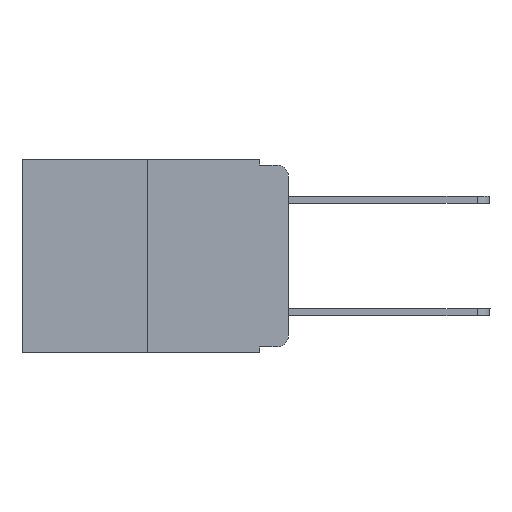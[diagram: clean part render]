
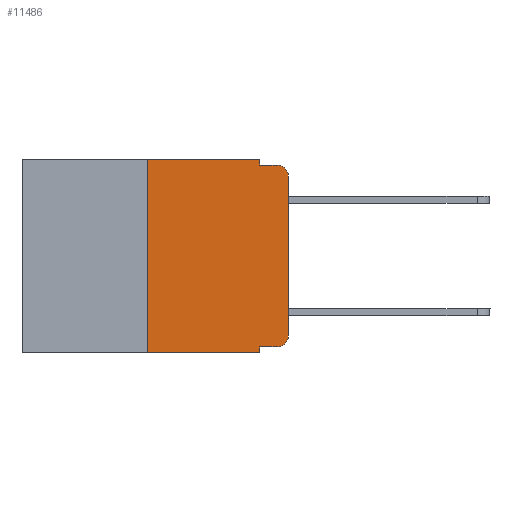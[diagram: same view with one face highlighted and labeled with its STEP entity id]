
A CAD part, left-side view. The second image highlights one B-rep face of the part: STEP entity #11486.
In plain terms, the highlighted planar face has unit normal (-1, 0, 0).
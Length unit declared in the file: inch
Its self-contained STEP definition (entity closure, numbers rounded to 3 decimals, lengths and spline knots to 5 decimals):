
#33 = DIRECTION ( 'NONE',  ( 0., 0., -1. ) ) ;
#128 = CARTESIAN_POINT ( 'NONE',  ( 0., 0.02, -0.01 ) ) ;
#131 = CARTESIAN_POINT ( 'NONE',  ( 0., 0., 0. ) ) ;
#171 = DIRECTION ( 'NONE',  ( 0., 0., 1. ) ) ;
#719 = CARTESIAN_POINT ( 'NONE',  ( 0., 0.473, -0.343 ) ) ;
#815 = DIRECTION ( 'NONE',  ( 1., 0., 0. ) ) ;
#1197 = CARTESIAN_POINT ( 'NONE',  ( 0., 0.051, -0.01 ) ) ;
#1289 = DIRECTION ( 'NONE',  ( 0., 0., -1. ) ) ;
#1542 = AXIS2_PLACEMENT_3D ( 'NONE', #11026, #815, #14529 ) ;
#1567 = EDGE_CURVE ( 'NONE', #2215, #2679, #11632, .T. ) ;
#1684 = EDGE_LOOP ( 'NONE', ( #5479, #13770, #14269, #2884, #1979, #5238, #12926, #9023, #13822, #14367 ) ) ;
#1750 = LINE ( 'NONE', #14259, #7792 ) ;
#1979 = ORIENTED_EDGE ( 'NONE', *, *, #6144, .F. ) ;
#2215 = VERTEX_POINT ( 'NONE', #10141 ) ;
#2273 = CARTESIAN_POINT ( 'NONE',  ( 0., 0.25, 0. ) ) ;
#2679 = VERTEX_POINT ( 'NONE', #8733 ) ;
#2732 = CARTESIAN_POINT ( 'NONE',  ( 0., 0.051, 0. ) ) ;
#2884 = ORIENTED_EDGE ( 'NONE', *, *, #7385, .F. ) ;
#3648 = CARTESIAN_POINT ( 'NONE',  ( 0., 0.051, -0.333 ) ) ;
#4303 = LINE ( 'NONE', #3648, #9275 ) ;
#4863 = CARTESIAN_POINT ( 'NONE',  ( 0., 0.02, -0.333 ) ) ;
#5002 = CARTESIAN_POINT ( 'NONE',  ( 0., 0.02, -0.313 ) ) ;
#5089 = LINE ( 'NONE', #9236, #8083 ) ;
#5238 = ORIENTED_EDGE ( 'NONE', *, *, #8038, .F. ) ;
#5258 = DIRECTION ( 'NONE',  ( 0., -1., 0. ) ) ;
#5479 = ORIENTED_EDGE ( 'NONE', *, *, #6393, .T. ) ;
#5553 = CARTESIAN_POINT ( 'NONE',  ( 0., 0.051, 0. ) ) ;
#5731 = DIRECTION ( 'NONE',  ( -1., 0., 0. ) ) ;
#5963 = CARTESIAN_POINT ( 'NONE',  ( 0., 0.25, -0.343 ) ) ;
#6144 = EDGE_CURVE ( 'NONE', #9274, #7700, #1750, .T. ) ;
#6151 = FACE_OUTER_BOUND ( 'NONE', #1684, .T. ) ;
#6393 = EDGE_CURVE ( 'NONE', #9495, #13925, #8878, .T. ) ;
#6537 = PLANE ( 'NONE',  #1542 ) ;
#6912 = CARTESIAN_POINT ( 'NONE',  ( 0., 0.02, -0.03 ) ) ;
#6970 = DIRECTION ( 'NONE',  ( 0., -1., 0. ) ) ;
#7385 = EDGE_CURVE ( 'NONE', #7700, #12518, #7408, .T. ) ;
#7408 = LINE ( 'NONE', #5553, #11868 ) ;
#7463 = DIRECTION ( 'NONE',  ( 0., -1., 0. ) ) ;
#7700 = VERTEX_POINT ( 'NONE', #2732 ) ;
#7792 = VECTOR ( 'NONE', #8607, 39.37008 ) ;
#7866 = VECTOR ( 'NONE', #33, 39.37008 ) ;
#8038 = EDGE_CURVE ( 'NONE', #13379, #9274, #5089, .T. ) ;
#8079 = DIRECTION ( 'NONE',  ( 0., 0., 1. ) ) ;
#8083 = VECTOR ( 'NONE', #171, 39.37008 ) ;
#8521 = DIRECTION ( 'NONE',  ( -1., 0., 0. ) ) ;
#8607 = DIRECTION ( 'NONE',  ( 0., -1., 0. ) ) ;
#8733 = CARTESIAN_POINT ( 'NONE',  ( 0., 0.051, -0.343 ) ) ;
#8878 = LINE ( 'NONE', #131, #10120 ) ;
#9023 = ORIENTED_EDGE ( 'NONE', *, *, #1567, .F. ) ;
#9236 = CARTESIAN_POINT ( 'NONE',  ( 0., 0.25, 0. ) ) ;
#9245 = CARTESIAN_POINT ( 'NONE',  ( 0., 0., -0.03 ) ) ;
#9274 = VERTEX_POINT ( 'NONE', #2273 ) ;
#9275 = VECTOR ( 'NONE', #6970, 39.37008 ) ;
#9476 = DIRECTION ( 'NONE',  ( 0., 0., -1. ) ) ;
#9495 = VERTEX_POINT ( 'NONE', #14291 ) ;
#9715 = CARTESIAN_POINT ( 'NONE',  ( 0., 0.051, -0.01 ) ) ;
#9999 = VERTEX_POINT ( 'NONE', #4863 ) ;
#10060 = EDGE_CURVE ( 'NONE', #9999, #9495, #10454, .T. ) ;
#10120 = VECTOR ( 'NONE', #8079, 39.37008 ) ;
#10141 = CARTESIAN_POINT ( 'NONE',  ( 0., 0.051, -0.333 ) ) ;
#10250 = VECTOR ( 'NONE', #5258, 39.37008 ) ;
#10418 = EDGE_CURVE ( 'NONE', #13925, #11175, #10641, .T. ) ;
#10454 = CIRCLE ( 'NONE', #12521, 0.02 ) ;
#10641 = CIRCLE ( 'NONE', #12131, 0.02 ) ;
#11026 = CARTESIAN_POINT ( 'NONE',  ( 0., 0.473, 0. ) ) ;
#11175 = VERTEX_POINT ( 'NONE', #128 ) ;
#11235 = DIRECTION ( 'NONE',  ( 0., 0., -1. ) ) ;
#11429 = EDGE_CURVE ( 'NONE', #13379, #2679, #12948, .T. ) ;
#11486 = ADVANCED_FACE ( 'NONE', ( #6151 ), #6537, .F. ) ;
#11632 = LINE ( 'NONE', #13694, #7866 ) ;
#11797 = VECTOR ( 'NONE', #7463, 39.37008 ) ;
#11868 = VECTOR ( 'NONE', #11235, 39.37008 ) ;
#12131 = AXIS2_PLACEMENT_3D ( 'NONE', #6912, #5731, #1289 ) ;
#12518 = VERTEX_POINT ( 'NONE', #1197 ) ;
#12521 = AXIS2_PLACEMENT_3D ( 'NONE', #5002, #8521, #9476 ) ;
#12926 = ORIENTED_EDGE ( 'NONE', *, *, #11429, .T. ) ;
#12948 = LINE ( 'NONE', #719, #10250 ) ;
#13068 = EDGE_CURVE ( 'NONE', #12518, #11175, #13612, .T. ) ;
#13379 = VERTEX_POINT ( 'NONE', #5963 ) ;
#13612 = LINE ( 'NONE', #9715, #11797 ) ;
#13694 = CARTESIAN_POINT ( 'NONE',  ( 0., 0.051, 0. ) ) ;
#13770 = ORIENTED_EDGE ( 'NONE', *, *, #10418, .T. ) ;
#13822 = ORIENTED_EDGE ( 'NONE', *, *, #14564, .T. ) ;
#13925 = VERTEX_POINT ( 'NONE', #9245 ) ;
#14259 = CARTESIAN_POINT ( 'NONE',  ( 0., 0.473, 0. ) ) ;
#14269 = ORIENTED_EDGE ( 'NONE', *, *, #13068, .F. ) ;
#14291 = CARTESIAN_POINT ( 'NONE',  ( 0., 0., -0.313 ) ) ;
#14367 = ORIENTED_EDGE ( 'NONE', *, *, #10060, .T. ) ;
#14529 = DIRECTION ( 'NONE',  ( 0., 0., -1. ) ) ;
#14564 = EDGE_CURVE ( 'NONE', #2215, #9999, #4303, .T. ) ;
